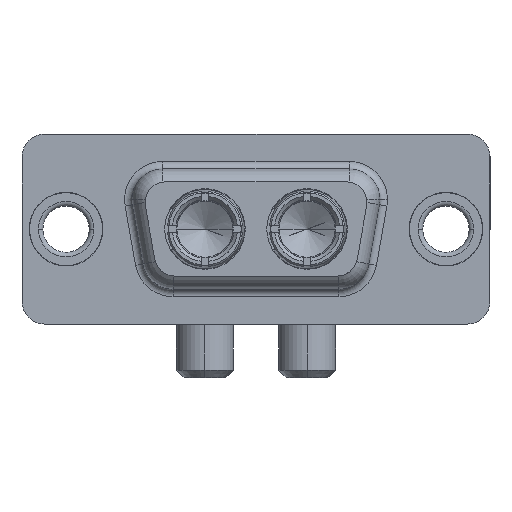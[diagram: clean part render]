
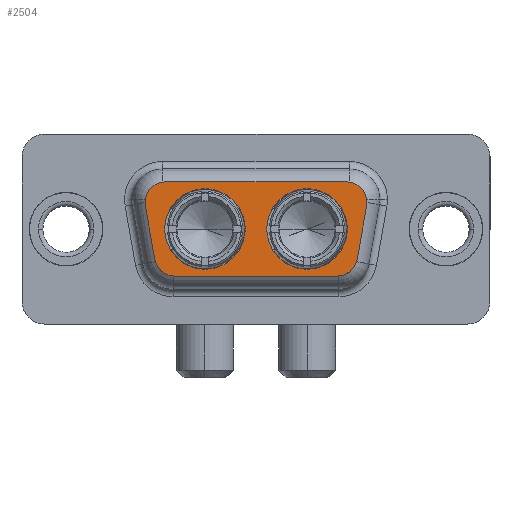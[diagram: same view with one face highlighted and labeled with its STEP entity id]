
A CAD part, top view. The second image highlights one B-rep face of the part: STEP entity #2504.
In plain terms, the highlighted planar face has unit normal (0, 0, 1).
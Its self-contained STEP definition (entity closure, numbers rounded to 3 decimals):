
#107 = CARTESIAN_POINT ( 'NONE',  ( 18.45, 3.1, 6.2 ) ) ;
#212 = VECTOR ( 'NONE', #455, 1000. ) ;
#237 = CIRCLE ( 'NONE', #5253, 1.35 ) ;
#322 = CIRCLE ( 'NONE', #8689, 1.35 ) ;
#347 = VERTEX_POINT ( 'NONE', #7735 ) ;
#385 = AXIS2_PLACEMENT_3D ( 'NONE', #4182, #6606, #9025 ) ;
#455 = DIRECTION ( 'NONE',  ( 0.174, -0.985, 0. ) ) ;
#505 = CARTESIAN_POINT ( 'NONE',  ( 17.833, -3.1, 6.2 ) ) ;
#569 = DIRECTION ( 'NONE',  ( 1., 0., 0. ) ) ;
#591 = ORIENTED_EDGE ( 'NONE', *, *, #7155, .T. ) ;
#609 = VERTEX_POINT ( 'NONE', #1733 ) ;
#729 = VERTEX_POINT ( 'NONE', #8494 ) ;
#800 = DIRECTION ( 'NONE',  ( 0., 0., 1. ) ) ;
#932 = DIRECTION ( 'NONE',  ( -1., 0., 0. ) ) ;
#936 = CARTESIAN_POINT ( 'NONE',  ( 17.833, -1.75, 6.2 ) ) ;
#1005 = ORIENTED_EDGE ( 'NONE', *, *, #6530, .T. ) ;
#1027 = EDGE_CURVE ( 'NONE', #3713, #347, #2497, .T. ) ;
#1075 = DIRECTION ( 'NONE',  ( 0., 0., 1. ) ) ;
#1091 = ORIENTED_EDGE ( 'NONE', *, *, #10086, .F. ) ;
#1094 = VERTEX_POINT ( 'NONE', #8019 ) ;
#1146 = CARTESIAN_POINT ( 'NONE',  ( 7.167, -3.1, 6.2 ) ) ;
#1331 = ORIENTED_EDGE ( 'NONE', *, *, #1027, .T. ) ;
#1353 = DIRECTION ( 'NONE',  ( 1., 0., 0. ) ) ;
#1462 = ORIENTED_EDGE ( 'NONE', *, *, #7311, .F. ) ;
#1607 = CARTESIAN_POINT ( 'NONE',  ( 19.779, 1.516, 6.2 ) ) ;
#1628 = AXIS2_PLACEMENT_3D ( 'NONE', #936, #2665, #4141 ) ;
#1644 = VECTOR ( 'NONE', #5234, 1000. ) ;
#1728 = CARTESIAN_POINT ( 'NONE',  ( 6.55, 3.1, 6.2 ) ) ;
#1733 = CARTESIAN_POINT ( 'NONE',  ( 6.55, 3.1, 6.2 ) ) ;
#2016 = DIRECTION ( 'NONE',  ( -1., 0., 0. ) ) ;
#2028 = CARTESIAN_POINT ( 'NONE',  ( 5.838, -1.984, 6.2 ) ) ;
#2111 = EDGE_LOOP ( 'NONE', ( #7566, #591, #1005, #1331, #6469, #3417, #7517, #7194, #10320 ) ) ;
#2133 = AXIS2_PLACEMENT_3D ( 'NONE', #3822, #7048, #1353 ) ;
#2193 = CARTESIAN_POINT ( 'NONE',  ( 6.49, 0., 6.2 ) ) ;
#2386 = EDGE_CURVE ( 'NONE', #1094, #6615, #237, .T. ) ;
#2458 = VERTEX_POINT ( 'NONE', #2853 ) ;
#2476 = VECTOR ( 'NONE', #4925, 1000. ) ;
#2497 = LINE ( 'NONE', #1607, #2476 ) ;
#2504 = ADVANCED_FACE ( 'NONE', ( #3694, #6917, #2801 ), #7660, .F. ) ;
#2665 = DIRECTION ( 'NONE',  ( 0., 0., 1. ) ) ;
#2797 = CARTESIAN_POINT ( 'NONE',  ( 5.221, 1.516, 6.2 ) ) ;
#2801 = FACE_OUTER_BOUND ( 'NONE', #2111, .T. ) ;
#2853 = CARTESIAN_POINT ( 'NONE',  ( 5.2, 1.75, 6.2 ) ) ;
#2904 = VERTEX_POINT ( 'NONE', #505 ) ;
#3034 = AXIS2_PLACEMENT_3D ( 'NONE', #8703, #7768, #569 ) ;
#3225 = CARTESIAN_POINT ( 'NONE',  ( 7.167, -1.75, 6.2 ) ) ;
#3317 = CIRCLE ( 'NONE', #4503, 2.65 ) ;
#3417 = ORIENTED_EDGE ( 'NONE', *, *, #8430, .T. ) ;
#3640 = AXIS2_PLACEMENT_3D ( 'NONE', #5958, #9867, #7558 ) ;
#3679 = VECTOR ( 'NONE', #932, 1000. ) ;
#3694 = FACE_BOUND ( 'NONE', #9590, .T. ) ;
#3707 = CARTESIAN_POINT ( 'NONE',  ( 19.162, -1.984, 6.2 ) ) ;
#3713 = VERTEX_POINT ( 'NONE', #3707 ) ;
#3822 = CARTESIAN_POINT ( 'NONE',  ( 15.86, 0., 6.2 ) ) ;
#3839 = CARTESIAN_POINT ( 'NONE',  ( 15.86, 0., 6.2 ) ) ;
#3891 = EDGE_CURVE ( 'NONE', #2458, #7142, #6402, .T. ) ;
#3913 = VERTEX_POINT ( 'NONE', #2193 ) ;
#4005 = CARTESIAN_POINT ( 'NONE',  ( 9.14, 0., 6.2 ) ) ;
#4141 = DIRECTION ( 'NONE',  ( -1., 0., 0. ) ) ;
#4182 = CARTESIAN_POINT ( 'NONE',  ( 9.14, 0., 6.2 ) ) ;
#4234 = ORIENTED_EDGE ( 'NONE', *, *, #7173, .F. ) ;
#4503 = AXIS2_PLACEMENT_3D ( 'NONE', #4005, #800, #5728 ) ;
#4870 = VERTEX_POINT ( 'NONE', #5723 ) ;
#4925 = DIRECTION ( 'NONE',  ( 0.174, 0.985, 0. ) ) ;
#4931 = LINE ( 'NONE', #1728, #3679 ) ;
#5130 = DIRECTION ( 'NONE',  ( -1., 0., 0. ) ) ;
#5185 = CARTESIAN_POINT ( 'NONE',  ( 7.167, -1.75, 6.2 ) ) ;
#5220 = EDGE_CURVE ( 'NONE', #609, #2458, #8172, .T. ) ;
#5227 = CIRCLE ( 'NONE', #385, 2.65 ) ;
#5234 = DIRECTION ( 'NONE',  ( 1., 0., 0. ) ) ;
#5253 = AXIS2_PLACEMENT_3D ( 'NONE', #3225, #9873, #7246 ) ;
#5581 = AXIS2_PLACEMENT_3D ( 'NONE', #5185, #10123, #5130 ) ;
#5672 = EDGE_CURVE ( 'NONE', #347, #8441, #322, .T. ) ;
#5723 = CARTESIAN_POINT ( 'NONE',  ( 11.79, 0., 6.2 ) ) ;
#5728 = DIRECTION ( 'NONE',  ( 1., 0., 0. ) ) ;
#5958 = CARTESIAN_POINT ( 'NONE',  ( 6.55, 1.75, 6.2 ) ) ;
#6149 = CIRCLE ( 'NONE', #1628, 1.35 ) ;
#6338 = EDGE_CURVE ( 'NONE', #729, #9814, #9532, .T. ) ;
#6402 = CIRCLE ( 'NONE', #3034, 1.35 ) ;
#6469 = ORIENTED_EDGE ( 'NONE', *, *, #5672, .T. ) ;
#6530 = EDGE_CURVE ( 'NONE', #2904, #3713, #6149, .T. ) ;
#6606 = DIRECTION ( 'NONE',  ( 0., 0., 1. ) ) ;
#6615 = VERTEX_POINT ( 'NONE', #1146 ) ;
#6717 = LINE ( 'NONE', #2028, #212 ) ;
#6760 = CARTESIAN_POINT ( 'NONE',  ( 18.45, 1.75, 6.2 ) ) ;
#6814 = DIRECTION ( 'NONE',  ( 0., 0., 1. ) ) ;
#6917 = FACE_BOUND ( 'NONE', #8463, .T. ) ;
#7017 = CIRCLE ( 'NONE', #9369, 2.65 ) ;
#7048 = DIRECTION ( 'NONE',  ( 0., 0., 1. ) ) ;
#7142 = VERTEX_POINT ( 'NONE', #2797 ) ;
#7155 = EDGE_CURVE ( 'NONE', #6615, #2904, #7897, .T. ) ;
#7173 = EDGE_CURVE ( 'NONE', #9814, #729, #7017, .T. ) ;
#7194 = ORIENTED_EDGE ( 'NONE', *, *, #3891, .T. ) ;
#7246 = DIRECTION ( 'NONE',  ( -1., 0., 0. ) ) ;
#7311 = EDGE_CURVE ( 'NONE', #3913, #4870, #3317, .T. ) ;
#7517 = ORIENTED_EDGE ( 'NONE', *, *, #5220, .T. ) ;
#7558 = DIRECTION ( 'NONE',  ( 1., 0., 0. ) ) ;
#7566 = ORIENTED_EDGE ( 'NONE', *, *, #2386, .T. ) ;
#7660 = PLANE ( 'NONE',  #5581 ) ;
#7666 = CARTESIAN_POINT ( 'NONE',  ( 18.51, 0., 6.2 ) ) ;
#7735 = CARTESIAN_POINT ( 'NONE',  ( 19.779, 1.516, 6.2 ) ) ;
#7768 = DIRECTION ( 'NONE',  ( 0., 0., 1. ) ) ;
#7897 = LINE ( 'NONE', #8329, #1644 ) ;
#8019 = CARTESIAN_POINT ( 'NONE',  ( 5.838, -1.984, 6.2 ) ) ;
#8172 = CIRCLE ( 'NONE', #3640, 1.35 ) ;
#8329 = CARTESIAN_POINT ( 'NONE',  ( 17.833, -3.1, 6.2 ) ) ;
#8430 = EDGE_CURVE ( 'NONE', #8441, #609, #4931, .T. ) ;
#8441 = VERTEX_POINT ( 'NONE', #107 ) ;
#8463 = EDGE_LOOP ( 'NONE', ( #1091, #1462 ) ) ;
#8494 = CARTESIAN_POINT ( 'NONE',  ( 13.21, 0., 6.2 ) ) ;
#8680 = DIRECTION ( 'NONE',  ( 1., 0., 0. ) ) ;
#8689 = AXIS2_PLACEMENT_3D ( 'NONE', #6760, #1075, #2016 ) ;
#8703 = CARTESIAN_POINT ( 'NONE',  ( 6.55, 1.75, 6.2 ) ) ;
#8942 = ORIENTED_EDGE ( 'NONE', *, *, #6338, .F. ) ;
#9025 = DIRECTION ( 'NONE',  ( 1., 0., 0. ) ) ;
#9369 = AXIS2_PLACEMENT_3D ( 'NONE', #3839, #6814, #8680 ) ;
#9532 = CIRCLE ( 'NONE', #2133, 2.65 ) ;
#9590 = EDGE_LOOP ( 'NONE', ( #4234, #8942 ) ) ;
#9814 = VERTEX_POINT ( 'NONE', #7666 ) ;
#9867 = DIRECTION ( 'NONE',  ( 0., 0., 1. ) ) ;
#9873 = DIRECTION ( 'NONE',  ( 0., 0., 1. ) ) ;
#10086 = EDGE_CURVE ( 'NONE', #4870, #3913, #5227, .T. ) ;
#10123 = DIRECTION ( 'NONE',  ( 0., 0., -1. ) ) ;
#10320 = ORIENTED_EDGE ( 'NONE', *, *, #10350, .T. ) ;
#10350 = EDGE_CURVE ( 'NONE', #7142, #1094, #6717, .T. ) ;
